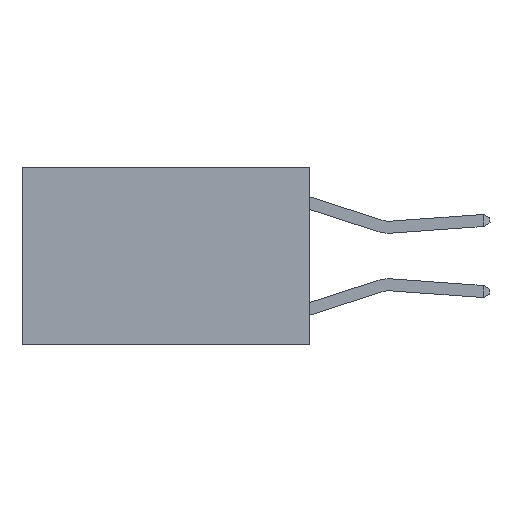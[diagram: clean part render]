
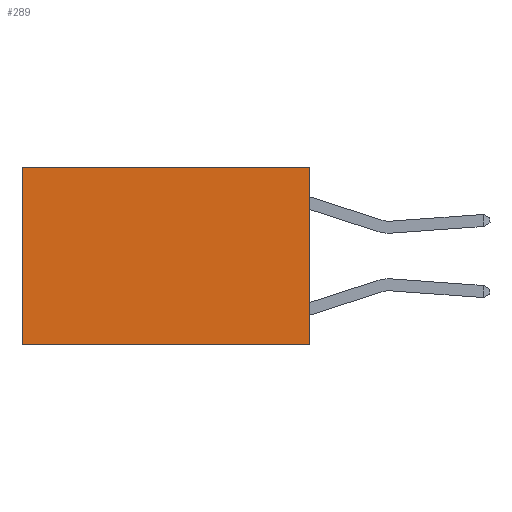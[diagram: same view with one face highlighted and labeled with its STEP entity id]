
A CAD part, left-side view. The second image highlights one B-rep face of the part: STEP entity #289.
In plain terms, the highlighted planar face has unit normal (-1, 0, 0).
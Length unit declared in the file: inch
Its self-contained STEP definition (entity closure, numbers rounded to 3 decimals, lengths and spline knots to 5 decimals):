
#289 = ADVANCED_FACE ( 'NONE', ( #16624 ), #11134, .F. ) ;
#809 = CARTESIAN_POINT ( 'NONE',  ( 0.2625, 0.6, 0. ) ) ;
#1290 = DIRECTION ( 'NONE',  ( 0., 0., -1. ) ) ;
#1487 = ORIENTED_EDGE ( 'NONE', *, *, #1770, .T. ) ;
#1770 = EDGE_CURVE ( 'NONE', #10043, #5874, #21560, .T. ) ;
#2497 = CARTESIAN_POINT ( 'NONE',  ( 0.2625, 0., -0.37 ) ) ;
#2539 = VECTOR ( 'NONE', #9788, 39.37008 ) ;
#2911 = EDGE_CURVE ( 'NONE', #5874, #16823, #22326, .T. ) ;
#3319 = VECTOR ( 'NONE', #19480, 39.37008 ) ;
#4408 = EDGE_LOOP ( 'NONE', ( #9022, #14271, #12994, #1487 ) ) ;
#5631 = LINE ( 'NONE', #2497, #9845 ) ;
#5801 = CARTESIAN_POINT ( 'NONE',  ( 0.2625, 0.6, 0. ) ) ;
#5874 = VERTEX_POINT ( 'NONE', #809 ) ;
#6645 = CARTESIAN_POINT ( 'NONE',  ( 0.2625, 0., -0.37 ) ) ;
#8260 = VECTOR ( 'NONE', #1290, 39.37008 ) ;
#8582 = AXIS2_PLACEMENT_3D ( 'NONE', #13621, #21631, #22753 ) ;
#9022 = ORIENTED_EDGE ( 'NONE', *, *, #2911, .T. ) ;
#9654 = EDGE_CURVE ( 'NONE', #10043, #22774, #15227, .T. ) ;
#9788 = DIRECTION ( 'NONE',  ( 0., 1., 0. ) ) ;
#9845 = VECTOR ( 'NONE', #16825, 39.37008 ) ;
#10043 = VERTEX_POINT ( 'NONE', #11264 ) ;
#10926 = CARTESIAN_POINT ( 'NONE',  ( 0.2625, 0., 0. ) ) ;
#11134 = PLANE ( 'NONE',  #8582 ) ;
#11264 = CARTESIAN_POINT ( 'NONE',  ( 0.2625, 0., 0. ) ) ;
#12994 = ORIENTED_EDGE ( 'NONE', *, *, #9654, .F. ) ;
#13621 = CARTESIAN_POINT ( 'NONE',  ( 0.2625, 0., 0. ) ) ;
#14271 = ORIENTED_EDGE ( 'NONE', *, *, #19815, .F. ) ;
#15227 = LINE ( 'NONE', #19120, #8260 ) ;
#16624 = FACE_OUTER_BOUND ( 'NONE', #4408, .T. ) ;
#16823 = VERTEX_POINT ( 'NONE', #19900 ) ;
#16825 = DIRECTION ( 'NONE',  ( 0., 1., 0. ) ) ;
#19120 = CARTESIAN_POINT ( 'NONE',  ( 0.2625, 0., 0. ) ) ;
#19480 = DIRECTION ( 'NONE',  ( 0., 0., -1. ) ) ;
#19815 = EDGE_CURVE ( 'NONE', #22774, #16823, #5631, .T. ) ;
#19900 = CARTESIAN_POINT ( 'NONE',  ( 0.2625, 0.6, -0.37 ) ) ;
#21560 = LINE ( 'NONE', #10926, #2539 ) ;
#21631 = DIRECTION ( 'NONE',  ( 1., 0., 0. ) ) ;
#22326 = LINE ( 'NONE', #5801, #3319 ) ;
#22753 = DIRECTION ( 'NONE',  ( 0., 0., -1. ) ) ;
#22774 = VERTEX_POINT ( 'NONE', #6645 ) ;
